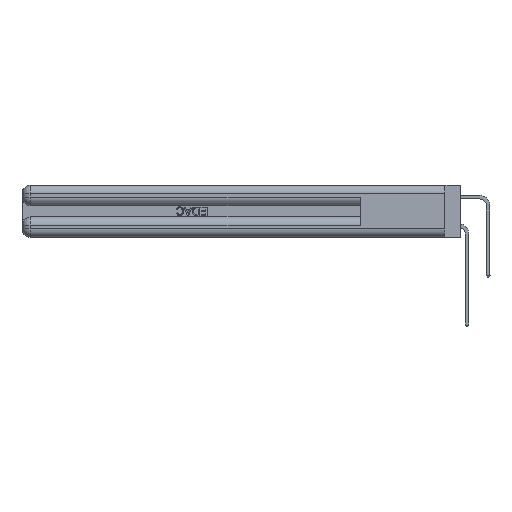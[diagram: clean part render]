
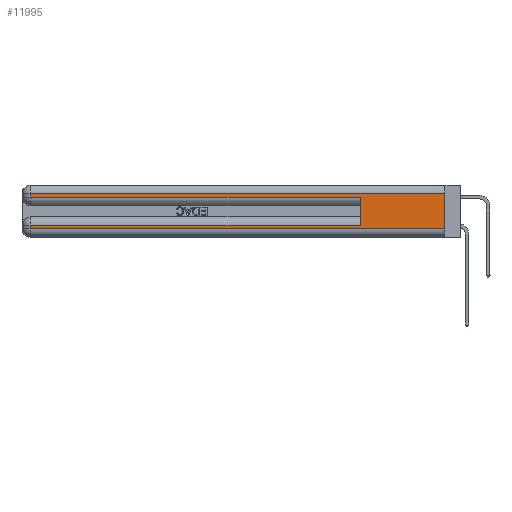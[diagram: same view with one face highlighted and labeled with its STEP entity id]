
A CAD part, left-side view. The second image highlights one B-rep face of the part: STEP entity #11995.
In plain terms, the highlighted planar face has unit normal (-1, 0, 0).
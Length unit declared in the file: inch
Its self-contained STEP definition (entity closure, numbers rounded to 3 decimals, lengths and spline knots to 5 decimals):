
#388 = FACE_OUTER_BOUND ( 'NONE', #21367, .T. ) ;
#438 = DIRECTION ( 'NONE',  ( 0., 0., -1. ) ) ;
#1403 = EDGE_CURVE ( 'NONE', #32703, #10326, #9212, .T. ) ;
#1483 = DIRECTION ( 'NONE',  ( 0., -1., 0. ) ) ;
#1579 = VERTEX_POINT ( 'NONE', #30681 ) ;
#2172 = VECTOR ( 'NONE', #2802, 39.37008 ) ;
#2802 = DIRECTION ( 'NONE',  ( 0., -1., 0. ) ) ;
#3589 = CARTESIAN_POINT ( 'NONE',  ( 0., 0., 0.31 ) ) ;
#4201 = AXIS2_PLACEMENT_3D ( 'NONE', #5674, #32279, #32555 ) ;
#4778 = LINE ( 'NONE', #29611, #16756 ) ;
#5303 = DIRECTION ( 'NONE',  ( 0., 1., 0. ) ) ;
#5674 = CARTESIAN_POINT ( 'NONE',  ( 0., 0., 0.37 ) ) ;
#6340 = LINE ( 'NONE', #16029, #2172 ) ;
#6667 = DIRECTION ( 'NONE',  ( 0., 0., 1. ) ) ;
#6828 = VECTOR ( 'NONE', #438, 39.37008 ) ;
#7038 = VERTEX_POINT ( 'NONE', #22812 ) ;
#8211 = CARTESIAN_POINT ( 'NONE',  ( 0., 0., 0.06 ) ) ;
#8825 = VECTOR ( 'NONE', #5303, 39.37008 ) ;
#9212 = LINE ( 'NONE', #8211, #39348 ) ;
#9862 = LINE ( 'NONE', #32998, #34323 ) ;
#10326 = VERTEX_POINT ( 'NONE', #24843 ) ;
#11079 = ORIENTED_EDGE ( 'NONE', *, *, #1403, .T. ) ;
#11721 = CARTESIAN_POINT ( 'NONE',  ( 0., 0., 0.085 ) ) ;
#11876 = ORIENTED_EDGE ( 'NONE', *, *, #17986, .T. ) ;
#11995 = ADVANCED_FACE ( 'NONE', ( #388 ), #29351, .F. ) ;
#13432 = DIRECTION ( 'NONE',  ( 0., 0., -1. ) ) ;
#14012 = EDGE_CURVE ( 'NONE', #32534, #1579, #26483, .T. ) ;
#14163 = VERTEX_POINT ( 'NONE', #29275 ) ;
#15098 = DIRECTION ( 'NONE',  ( 0., 0., -1. ) ) ;
#16029 = CARTESIAN_POINT ( 'NONE',  ( 0., 0., 0.285 ) ) ;
#16373 = LINE ( 'NONE', #29575, #33038 ) ;
#16756 = VECTOR ( 'NONE', #19712, 39.37008 ) ;
#17113 = EDGE_CURVE ( 'NONE', #33780, #10326, #16373, .T. ) ;
#17898 = ORIENTED_EDGE ( 'NONE', *, *, #19126, .T. ) ;
#17986 = EDGE_CURVE ( 'NONE', #32745, #7038, #19914, .T. ) ;
#18336 = EDGE_CURVE ( 'NONE', #33780, #32745, #4778, .T. ) ;
#19110 = ORIENTED_EDGE ( 'NONE', *, *, #17113, .F. ) ;
#19126 = EDGE_CURVE ( 'NONE', #1579, #32703, #24515, .T. ) ;
#19712 = DIRECTION ( 'NONE',  ( 0., 1., 0. ) ) ;
#19914 = LINE ( 'NONE', #21216, #31360 ) ;
#21127 = CARTESIAN_POINT ( 'NONE',  ( 0., 2.94, 0.06 ) ) ;
#21216 = CARTESIAN_POINT ( 'NONE',  ( 0., 2.94, 0.37 ) ) ;
#21367 = EDGE_LOOP ( 'NONE', ( #19110, #25039, #11876, #26656, #38859, #35915, #17898, #11079 ) ) ;
#22812 = CARTESIAN_POINT ( 'NONE',  ( 0., 2.94, 0.285 ) ) ;
#24515 = LINE ( 'NONE', #40815, #6828 ) ;
#24843 = CARTESIAN_POINT ( 'NONE',  ( 0., 0., 0.06 ) ) ;
#25039 = ORIENTED_EDGE ( 'NONE', *, *, #18336, .T. ) ;
#26483 = LINE ( 'NONE', #11721, #8825 ) ;
#26656 = ORIENTED_EDGE ( 'NONE', *, *, #36472, .T. ) ;
#29275 = CARTESIAN_POINT ( 'NONE',  ( 0., 0.6, 0.285 ) ) ;
#29351 = PLANE ( 'NONE',  #4201 ) ;
#29575 = CARTESIAN_POINT ( 'NONE',  ( 0., 0., 0.37 ) ) ;
#29611 = CARTESIAN_POINT ( 'NONE',  ( 0., 0., 0.31 ) ) ;
#30294 = CARTESIAN_POINT ( 'NONE',  ( 0., 0.6, 0.085 ) ) ;
#30681 = CARTESIAN_POINT ( 'NONE',  ( 0., 2.94, 0.085 ) ) ;
#31307 = CARTESIAN_POINT ( 'NONE',  ( 0., 2.94, 0.31 ) ) ;
#31360 = VECTOR ( 'NONE', #15098, 39.37008 ) ;
#32279 = DIRECTION ( 'NONE',  ( 1., 0., 0. ) ) ;
#32534 = VERTEX_POINT ( 'NONE', #30294 ) ;
#32555 = DIRECTION ( 'NONE',  ( 0., 0., -1. ) ) ;
#32703 = VERTEX_POINT ( 'NONE', #21127 ) ;
#32745 = VERTEX_POINT ( 'NONE', #31307 ) ;
#32998 = CARTESIAN_POINT ( 'NONE',  ( 0., 0.6, 0.145 ) ) ;
#33038 = VECTOR ( 'NONE', #13432, 39.37008 ) ;
#33780 = VERTEX_POINT ( 'NONE', #3589 ) ;
#34323 = VECTOR ( 'NONE', #6667, 39.37008 ) ;
#35915 = ORIENTED_EDGE ( 'NONE', *, *, #14012, .T. ) ;
#36472 = EDGE_CURVE ( 'NONE', #7038, #14163, #6340, .T. ) ;
#38764 = EDGE_CURVE ( 'NONE', #32534, #14163, #9862, .T. ) ;
#38859 = ORIENTED_EDGE ( 'NONE', *, *, #38764, .F. ) ;
#39348 = VECTOR ( 'NONE', #1483, 39.37008 ) ;
#40815 = CARTESIAN_POINT ( 'NONE',  ( 0., 2.94, 0.37 ) ) ;
